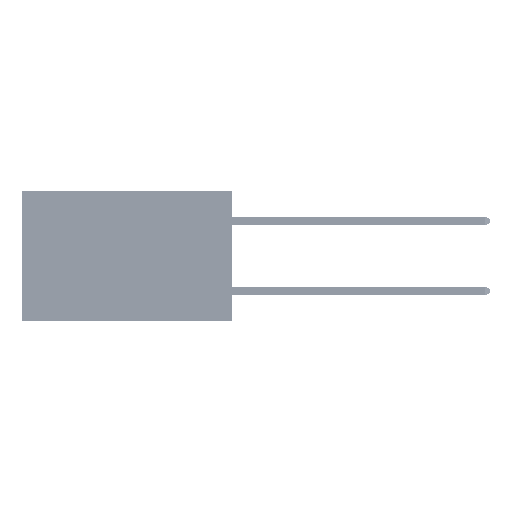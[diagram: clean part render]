
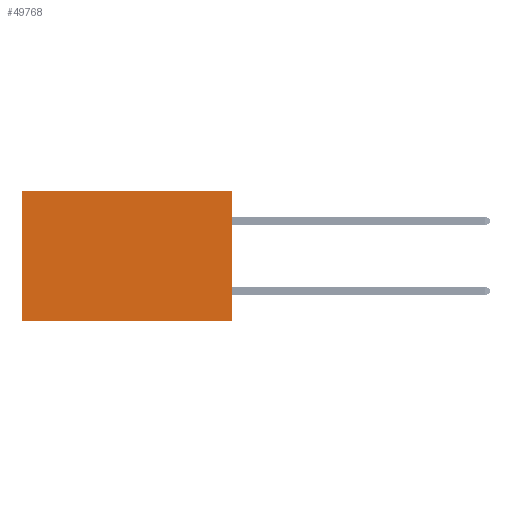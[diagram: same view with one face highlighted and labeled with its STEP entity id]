
A CAD part, left-side view. The second image highlights one B-rep face of the part: STEP entity #49768.
In plain terms, the highlighted planar face has unit normal (-1, 0, 0).
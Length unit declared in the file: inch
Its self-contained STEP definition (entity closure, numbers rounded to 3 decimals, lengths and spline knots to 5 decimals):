
#1218 = LINE ( 'NONE', #35616, #26409 ) ;
#2475 = EDGE_CURVE ( 'NONE', #18855, #36195, #14635, .T. ) ;
#2845 = PLANE ( 'NONE',  #14411 ) ;
#4737 = ORIENTED_EDGE ( 'NONE', *, *, #17793, .F. ) ;
#5783 = CARTESIAN_POINT ( 'NONE',  ( 0.2875, 0., 0. ) ) ;
#7063 = EDGE_CURVE ( 'NONE', #18855, #12114, #47602, .T. ) ;
#7536 = CARTESIAN_POINT ( 'NONE',  ( 0.2875, 0., -0.37 ) ) ;
#9502 = CARTESIAN_POINT ( 'NONE',  ( 0.2875, 0.6, 0. ) ) ;
#12114 = VERTEX_POINT ( 'NONE', #9502 ) ;
#13057 = VECTOR ( 'NONE', #22270, 39.37008 ) ;
#14411 = AXIS2_PLACEMENT_3D ( 'NONE', #23209, #39760, #27282 ) ;
#14635 = LINE ( 'NONE', #35476, #37951 ) ;
#17131 = EDGE_LOOP ( 'NONE', ( #46606, #4737, #18791, #21168 ) ) ;
#17793 = EDGE_CURVE ( 'NONE', #36195, #26949, #1218, .T. ) ;
#18791 = ORIENTED_EDGE ( 'NONE', *, *, #2475, .F. ) ;
#18855 = VERTEX_POINT ( 'NONE', #5783 ) ;
#18861 = EDGE_CURVE ( 'NONE', #12114, #26949, #49659, .T. ) ;
#21168 = ORIENTED_EDGE ( 'NONE', *, *, #7063, .T. ) ;
#22270 = DIRECTION ( 'NONE',  ( 0., 0., -1. ) ) ;
#23209 = CARTESIAN_POINT ( 'NONE',  ( 0.2875, 0., 0. ) ) ;
#24969 = CARTESIAN_POINT ( 'NONE',  ( 0.2875, 0.6, -0.37 ) ) ;
#26010 = CARTESIAN_POINT ( 'NONE',  ( 0.2875, 0.6, 0. ) ) ;
#26409 = VECTOR ( 'NONE', #39649, 39.37008 ) ;
#26949 = VERTEX_POINT ( 'NONE', #24969 ) ;
#27282 = DIRECTION ( 'NONE',  ( 0., 0., -1. ) ) ;
#29915 = VECTOR ( 'NONE', #42889, 39.37008 ) ;
#30358 = CARTESIAN_POINT ( 'NONE',  ( 0.2875, 0., 0. ) ) ;
#35476 = CARTESIAN_POINT ( 'NONE',  ( 0.2875, 0., 0. ) ) ;
#35616 = CARTESIAN_POINT ( 'NONE',  ( 0.2875, 0., -0.37 ) ) ;
#36195 = VERTEX_POINT ( 'NONE', #7536 ) ;
#37553 = FACE_OUTER_BOUND ( 'NONE', #17131, .T. ) ;
#37951 = VECTOR ( 'NONE', #47835, 39.37008 ) ;
#39649 = DIRECTION ( 'NONE',  ( 0., 1., 0. ) ) ;
#39760 = DIRECTION ( 'NONE',  ( 1., 0., 0. ) ) ;
#42889 = DIRECTION ( 'NONE',  ( 0., 1., 0. ) ) ;
#46606 = ORIENTED_EDGE ( 'NONE', *, *, #18861, .T. ) ;
#47602 = LINE ( 'NONE', #30358, #29915 ) ;
#47835 = DIRECTION ( 'NONE',  ( 0., 0., -1. ) ) ;
#49659 = LINE ( 'NONE', #26010, #13057 ) ;
#49768 = ADVANCED_FACE ( 'NONE', ( #37553 ), #2845, .F. ) ;
